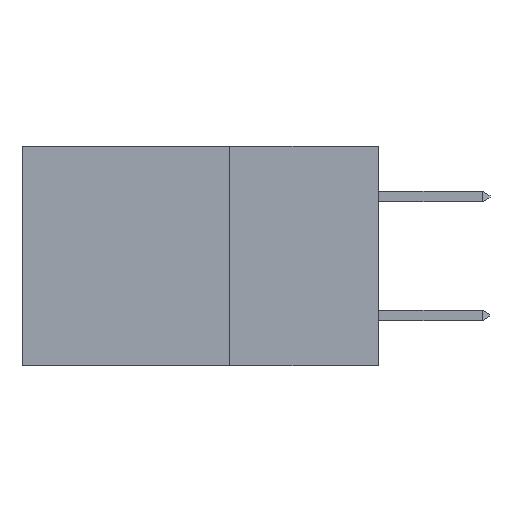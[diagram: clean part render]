
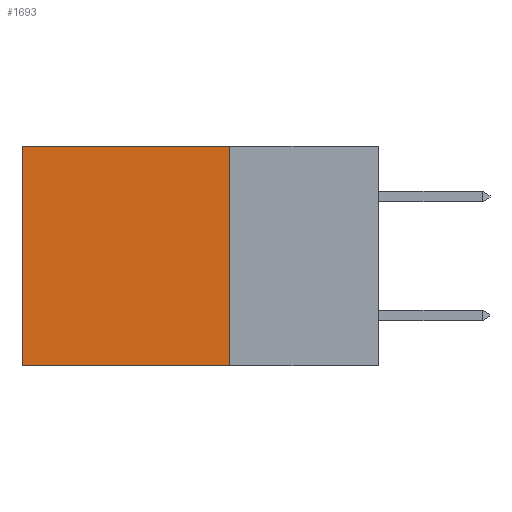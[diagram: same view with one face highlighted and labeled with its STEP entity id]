
A CAD part, left-side view. The second image highlights one B-rep face of the part: STEP entity #1693.
In plain terms, the highlighted planar face has unit normal (-1, 0, 0).
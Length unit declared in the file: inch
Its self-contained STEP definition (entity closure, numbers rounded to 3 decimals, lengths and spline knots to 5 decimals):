
#1103 = EDGE_CURVE ( 'NONE', #10067, #7145, #2957, .T. ) ;
#1565 = EDGE_CURVE ( 'NONE', #10067, #6714, #9906, .T. ) ;
#1646 = ORIENTED_EDGE ( 'NONE', *, *, #2862, .T. ) ;
#1693 = ADVANCED_FACE ( 'NONE', ( #8565 ), #2951, .F. ) ;
#2382 = CARTESIAN_POINT ( 'NONE',  ( 0.298, 0.6, 0. ) ) ;
#2862 = EDGE_CURVE ( 'NONE', #7145, #8441, #3312, .T. ) ;
#2951 = PLANE ( 'NONE',  #6566 ) ;
#2957 = LINE ( 'NONE', #7389, #7090 ) ;
#3116 = CARTESIAN_POINT ( 'NONE',  ( 0.298, 0.25, 0. ) ) ;
#3312 = LINE ( 'NONE', #2382, #7420 ) ;
#3605 = CARTESIAN_POINT ( 'NONE',  ( 0.298, 0.6, 0. ) ) ;
#3690 = DIRECTION ( 'NONE',  ( 0., 0., -1. ) ) ;
#3951 = ORIENTED_EDGE ( 'NONE', *, *, #4607, .F. ) ;
#4332 = CARTESIAN_POINT ( 'NONE',  ( 0.298, 0.6, -0.37 ) ) ;
#4607 = EDGE_CURVE ( 'NONE', #6714, #8441, #7479, .T. ) ;
#4718 = CARTESIAN_POINT ( 'NONE',  ( 0.298, 0.25, -0.37 ) ) ;
#4888 = CARTESIAN_POINT ( 'NONE',  ( 0.298, 0.25, -0.37 ) ) ;
#5175 = CARTESIAN_POINT ( 'NONE',  ( 0.298, 0.25, 0. ) ) ;
#5176 = DIRECTION ( 'NONE',  ( 0., 0., -1. ) ) ;
#5469 = VECTOR ( 'NONE', #7973, 39.37008 ) ;
#5593 = EDGE_LOOP ( 'NONE', ( #1646, #3951, #7923, #8164 ) ) ;
#5987 = DIRECTION ( 'NONE',  ( 1., 0., 0. ) ) ;
#6478 = DIRECTION ( 'NONE',  ( 0., 0., -1. ) ) ;
#6566 = AXIS2_PLACEMENT_3D ( 'NONE', #3116, #5987, #5176 ) ;
#6714 = VERTEX_POINT ( 'NONE', #4718 ) ;
#7090 = VECTOR ( 'NONE', #7381, 39.37008 ) ;
#7145 = VERTEX_POINT ( 'NONE', #3605 ) ;
#7381 = DIRECTION ( 'NONE',  ( 0., 1., 0. ) ) ;
#7389 = CARTESIAN_POINT ( 'NONE',  ( 0.298, 0.25, 0. ) ) ;
#7420 = VECTOR ( 'NONE', #3690, 39.37008 ) ;
#7479 = LINE ( 'NONE', #4888, #5469 ) ;
#7923 = ORIENTED_EDGE ( 'NONE', *, *, #1565, .F. ) ;
#7973 = DIRECTION ( 'NONE',  ( 0., 1., 0. ) ) ;
#8009 = VECTOR ( 'NONE', #6478, 39.37008 ) ;
#8164 = ORIENTED_EDGE ( 'NONE', *, *, #1103, .T. ) ;
#8441 = VERTEX_POINT ( 'NONE', #4332 ) ;
#8565 = FACE_OUTER_BOUND ( 'NONE', #5593, .T. ) ;
#8738 = CARTESIAN_POINT ( 'NONE',  ( 0.298, 0.25, 0. ) ) ;
#9906 = LINE ( 'NONE', #5175, #8009 ) ;
#10067 = VERTEX_POINT ( 'NONE', #8738 ) ;
